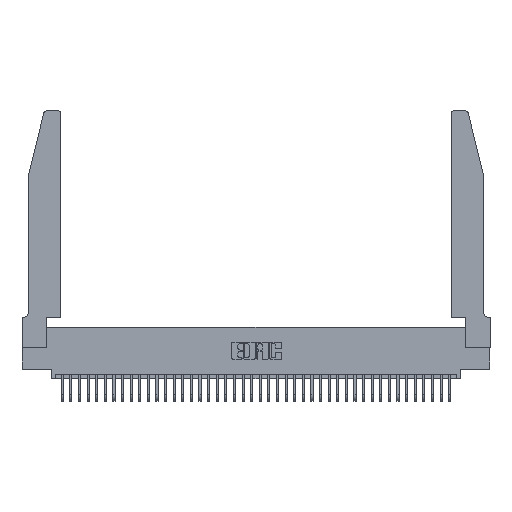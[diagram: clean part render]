
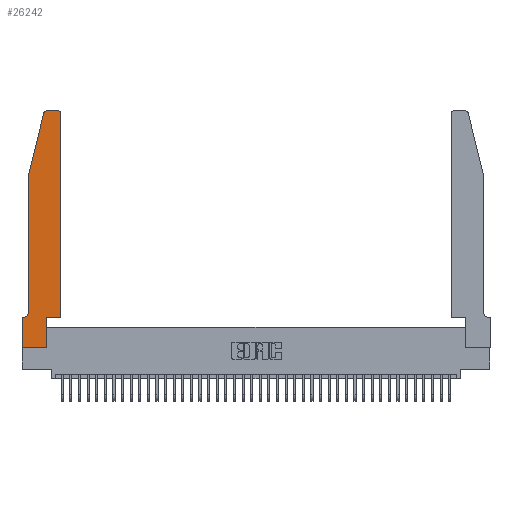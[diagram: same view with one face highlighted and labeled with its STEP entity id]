
A CAD part, top view. The second image highlights one B-rep face of the part: STEP entity #26242.
In plain terms, the highlighted planar face has unit normal (0, 0, 1).
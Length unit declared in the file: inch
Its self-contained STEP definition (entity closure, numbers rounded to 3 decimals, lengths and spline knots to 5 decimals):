
#893 = DIRECTION ( 'NONE',  ( 0., -1., 0. ) ) ;
#2087 = CARTESIAN_POINT ( 'NONE',  ( 0.0055, 0.42, 0.37 ) ) ;
#2613 = DIRECTION ( 'NONE',  ( 1., 0., 0. ) ) ;
#2983 = VECTOR ( 'NONE', #22376, 39.37008 ) ;
#3401 = CARTESIAN_POINT ( 'NONE',  ( 0.4505, 0.35, 0.37 ) ) ;
#3500 = EDGE_CURVE ( 'NONE', #4464, #25089, #34095, .T. ) ;
#4464 = VERTEX_POINT ( 'NONE', #4735 ) ;
#4735 = CARTESIAN_POINT ( 'NONE',  ( 0., 0., 0.37 ) ) ;
#4851 = EDGE_CURVE ( 'NONE', #22311, #32919, #14984, .T. ) ;
#5073 = DIRECTION ( 'NONE',  ( -1., 0., 0. ) ) ;
#5286 = CARTESIAN_POINT ( 'NONE',  ( 0.0055, 0.35, 0.37 ) ) ;
#5504 = ORIENTED_EDGE ( 'NONE', *, *, #19682, .T. ) ;
#5599 = DIRECTION ( 'NONE',  ( 0., -1., 0. ) ) ;
#5680 = CARTESIAN_POINT ( 'NONE',  ( 0.2865, 0., 0.37 ) ) ;
#6239 = EDGE_CURVE ( 'NONE', #14895, #22311, #21982, .T. ) ;
#7033 = VECTOR ( 'NONE', #27656, 39.37008 ) ;
#7586 = ORIENTED_EDGE ( 'NONE', *, *, #30416, .T. ) ;
#7809 = EDGE_CURVE ( 'NONE', #32919, #4464, #17133, .T. ) ;
#8816 = ORIENTED_EDGE ( 'NONE', *, *, #16956, .T. ) ;
#9170 = CARTESIAN_POINT ( 'NONE',  ( 0.4205, 2.72, 0.37 ) ) ;
#9258 = AXIS2_PLACEMENT_3D ( 'NONE', #38677, #20594, #2613 ) ;
#9337 = CARTESIAN_POINT ( 'NONE',  ( 0.2865, 0.35, 0.37 ) ) ;
#10950 = LINE ( 'NONE', #18846, #27995 ) ;
#11729 = CARTESIAN_POINT ( 'NONE',  ( 0., 0., 0.37 ) ) ;
#11817 = CARTESIAN_POINT ( 'NONE',  ( 0.284, 2.75, 0.37 ) ) ;
#11835 = VECTOR ( 'NONE', #20979, 39.37008 ) ;
#12016 = DIRECTION ( 'NONE',  ( 0., 0., 1. ) ) ;
#12177 = DIRECTION ( 'NONE',  ( 1., 0., 0. ) ) ;
#13197 = ORIENTED_EDGE ( 'NONE', *, *, #34778, .T. ) ;
#13414 = VERTEX_POINT ( 'NONE', #24018 ) ;
#14557 = CIRCLE ( 'NONE', #21617, 0.03 ) ;
#14716 = ORIENTED_EDGE ( 'NONE', *, *, #6239, .T. ) ;
#14719 = ORIENTED_EDGE ( 'NONE', *, *, #37024, .T. ) ;
#14895 = VERTEX_POINT ( 'NONE', #34263 ) ;
#14984 = LINE ( 'NONE', #21560, #7033 ) ;
#14992 = CARTESIAN_POINT ( 'NONE',  ( 0.0755, 2., 0.37 ) ) ;
#15371 = DIRECTION ( 'NONE',  ( 0., 1., 0. ) ) ;
#15422 = VERTEX_POINT ( 'NONE', #27723 ) ;
#15511 = VERTEX_POINT ( 'NONE', #28498 ) ;
#16713 = FACE_OUTER_BOUND ( 'NONE', #32721, .T. ) ;
#16956 = EDGE_CURVE ( 'NONE', #25142, #20718, #32447, .T. ) ;
#17133 = LINE ( 'NONE', #11729, #32326 ) ;
#18846 = CARTESIAN_POINT ( 'NONE',  ( 0.0755, 2., 0.37 ) ) ;
#19682 = EDGE_CURVE ( 'NONE', #29112, #14895, #10950, .T. ) ;
#20060 = ORIENTED_EDGE ( 'NONE', *, *, #3500, .T. ) ;
#20594 = DIRECTION ( 'NONE',  ( 0., 0., 1. ) ) ;
#20599 = DIRECTION ( 'NONE',  ( 1., 0., 0. ) ) ;
#20718 = VERTEX_POINT ( 'NONE', #26331 ) ;
#20937 = CARTESIAN_POINT ( 'NONE',  ( 0.2605, 2.75, 0.37 ) ) ;
#20979 = DIRECTION ( 'NONE',  ( 1., 0., 0. ) ) ;
#21560 = CARTESIAN_POINT ( 'NONE',  ( 0.0755, 0.35, 0.37 ) ) ;
#21617 = AXIS2_PLACEMENT_3D ( 'NONE', #9170, #30314, #12177 ) ;
#21982 = CIRCLE ( 'NONE', #28985, 0.07 ) ;
#22311 = VERTEX_POINT ( 'NONE', #5286 ) ;
#22376 = DIRECTION ( 'NONE',  ( -0.239, -0.971, 0. ) ) ;
#22575 = LINE ( 'NONE', #38682, #30687 ) ;
#23085 = DIRECTION ( 'NONE',  ( 0., 0., -1. ) ) ;
#23984 = DIRECTION ( 'NONE',  ( -1., 0., 0. ) ) ;
#24018 = CARTESIAN_POINT ( 'NONE',  ( 0.4505, 0.35, 0.37 ) ) ;
#25089 = VERTEX_POINT ( 'NONE', #5680 ) ;
#25142 = VERTEX_POINT ( 'NONE', #11817 ) ;
#25225 = VERTEX_POINT ( 'NONE', #9337 ) ;
#25418 = CARTESIAN_POINT ( 'NONE',  ( 0.0755, 2., 0.37 ) ) ;
#26242 = ADVANCED_FACE ( 'NONE', ( #16713 ), #35550, .T. ) ;
#26331 = CARTESIAN_POINT ( 'NONE',  ( 0.25487, 2.72718, 0.37 ) ) ;
#26354 = LINE ( 'NONE', #30501, #33485 ) ;
#27065 = ORIENTED_EDGE ( 'NONE', *, *, #7809, .T. ) ;
#27487 = DIRECTION ( 'NONE',  ( 0., 1., 0. ) ) ;
#27656 = DIRECTION ( 'NONE',  ( -1., 0., 0. ) ) ;
#27723 = CARTESIAN_POINT ( 'NONE',  ( 0.4505, 2.72, 0.37 ) ) ;
#27995 = VECTOR ( 'NONE', #893, 39.37008 ) ;
#28498 = CARTESIAN_POINT ( 'NONE',  ( 0.4205, 2.75, 0.37 ) ) ;
#28985 = AXIS2_PLACEMENT_3D ( 'NONE', #2087, #23085, #5073 ) ;
#29096 = ORIENTED_EDGE ( 'NONE', *, *, #36634, .T. ) ;
#29112 = VERTEX_POINT ( 'NONE', #14992 ) ;
#29240 = VECTOR ( 'NONE', #27487, 39.37008 ) ;
#30156 = CARTESIAN_POINT ( 'NONE',  ( 0.284, 2.72, 0.37 ) ) ;
#30314 = DIRECTION ( 'NONE',  ( 0., 0., 1. ) ) ;
#30416 = EDGE_CURVE ( 'NONE', #13414, #15422, #37282, .T. ) ;
#30501 = CARTESIAN_POINT ( 'NONE',  ( 0.2865, 0.35, 0.37 ) ) ;
#30687 = VECTOR ( 'NONE', #20599, 39.37008 ) ;
#30991 = EDGE_CURVE ( 'NONE', #25089, #25225, #26354, .T. ) ;
#32326 = VECTOR ( 'NONE', #5599, 39.37008 ) ;
#32447 = CIRCLE ( 'NONE', #35294, 0.03 ) ;
#32700 = VECTOR ( 'NONE', #23984, 39.37008 ) ;
#32721 = EDGE_LOOP ( 'NONE', ( #33387, #8816, #13197, #5504, #14716, #38262, #27065, #20060, #36305, #14719, #7586, #29096 ) ) ;
#32919 = VERTEX_POINT ( 'NONE', #36953 ) ;
#33199 = DIRECTION ( 'NONE',  ( 1., 0., 0. ) ) ;
#33387 = ORIENTED_EDGE ( 'NONE', *, *, #34596, .T. ) ;
#33485 = VECTOR ( 'NONE', #15371, 39.37008 ) ;
#33657 = LINE ( 'NONE', #20937, #32700 ) ;
#34095 = LINE ( 'NONE', #39071, #11835 ) ;
#34263 = CARTESIAN_POINT ( 'NONE',  ( 0.0755, 0.42, 0.37 ) ) ;
#34596 = EDGE_CURVE ( 'NONE', #15511, #25142, #33657, .T. ) ;
#34778 = EDGE_CURVE ( 'NONE', #20718, #29112, #37849, .T. ) ;
#35294 = AXIS2_PLACEMENT_3D ( 'NONE', #30156, #12016, #33199 ) ;
#35550 = PLANE ( 'NONE',  #9258 ) ;
#36305 = ORIENTED_EDGE ( 'NONE', *, *, #30991, .T. ) ;
#36634 = EDGE_CURVE ( 'NONE', #15422, #15511, #14557, .T. ) ;
#36953 = CARTESIAN_POINT ( 'NONE',  ( 0., 0.35, 0.37 ) ) ;
#37024 = EDGE_CURVE ( 'NONE', #25225, #13414, #22575, .T. ) ;
#37282 = LINE ( 'NONE', #3401, #29240 ) ;
#37849 = LINE ( 'NONE', #25418, #2983 ) ;
#38262 = ORIENTED_EDGE ( 'NONE', *, *, #4851, .T. ) ;
#38677 = CARTESIAN_POINT ( 'NONE',  ( 0., 0.35, 0.37 ) ) ;
#38682 = CARTESIAN_POINT ( 'NONE',  ( 0.4505, 0.35, 0.37 ) ) ;
#39071 = CARTESIAN_POINT ( 'NONE',  ( 0., 0., 0.37 ) ) ;
